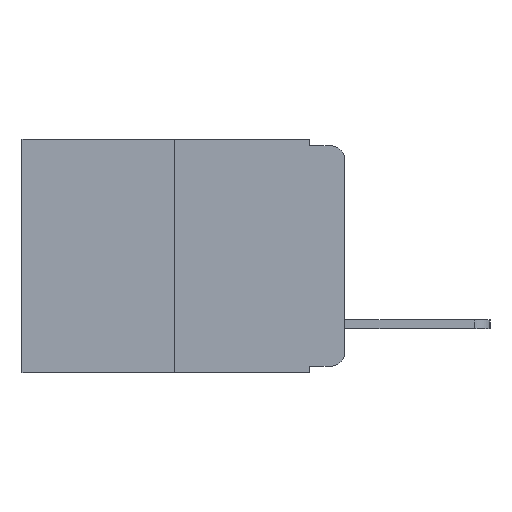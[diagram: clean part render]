
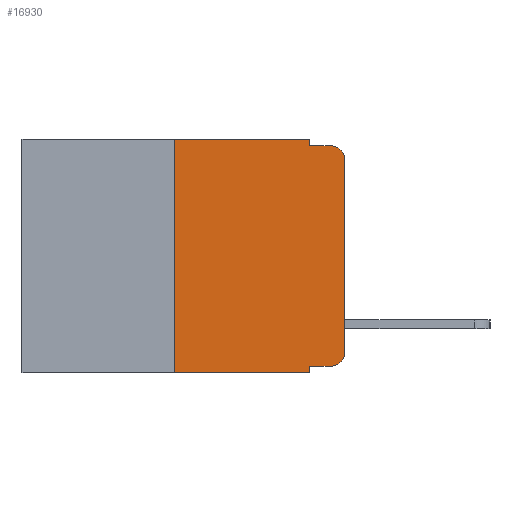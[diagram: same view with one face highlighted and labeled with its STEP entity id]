
A CAD part, left-side view. The second image highlights one B-rep face of the part: STEP entity #16930.
In plain terms, the highlighted planar face has unit normal (-1, 0, 0).
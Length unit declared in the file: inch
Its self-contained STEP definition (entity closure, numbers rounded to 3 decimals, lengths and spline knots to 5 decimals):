
#282 = ORIENTED_EDGE ( 'NONE', *, *, #3783, .F. ) ;
#1372 = DIRECTION ( 'NONE',  ( -1., 0., 0. ) ) ;
#2308 = VERTEX_POINT ( 'NONE', #12638 ) ;
#2593 = DIRECTION ( 'NONE',  ( 0., 0., -1. ) ) ;
#2771 = AXIS2_PLACEMENT_3D ( 'NONE', #6258, #17413, #7916 ) ;
#2850 = ORIENTED_EDGE ( 'NONE', *, *, #12250, .F. ) ;
#3260 = VECTOR ( 'NONE', #17030, 39.37008 ) ;
#3479 = DIRECTION ( 'NONE',  ( 0., -1., 0. ) ) ;
#3717 = CARTESIAN_POINT ( 'NONE',  ( 0., 0.051, 0. ) ) ;
#3783 = EDGE_CURVE ( 'NONE', #11301, #4717, #6162, .T. ) ;
#4101 = CIRCLE ( 'NONE', #8152, 0.02 ) ;
#4219 = CARTESIAN_POINT ( 'NONE',  ( 0., 0.051, -0.333 ) ) ;
#4538 = VECTOR ( 'NONE', #3479, 39.37008 ) ;
#4717 = VERTEX_POINT ( 'NONE', #18378 ) ;
#5120 = ORIENTED_EDGE ( 'NONE', *, *, #14346, .F. ) ;
#5604 = EDGE_CURVE ( 'NONE', #2308, #9613, #17796, .T. ) ;
#5658 = CARTESIAN_POINT ( 'NONE',  ( 0., 0.051, -0.01 ) ) ;
#5684 = CARTESIAN_POINT ( 'NONE',  ( 0., 0.051, 0. ) ) ;
#6162 = LINE ( 'NONE', #19746, #17871 ) ;
#6258 = CARTESIAN_POINT ( 'NONE',  ( 0., 0.02, -0.313 ) ) ;
#6442 = VERTEX_POINT ( 'NONE', #6681 ) ;
#6450 = LINE ( 'NONE', #9132, #6989 ) ;
#6535 = EDGE_LOOP ( 'NONE', ( #10719, #15408, #20553, #16887, #282, #5120, #18838, #2850, #7184, #16151 ) ) ;
#6622 = DIRECTION ( 'NONE',  ( 0., 0., 1. ) ) ;
#6681 = CARTESIAN_POINT ( 'NONE',  ( 0., 0.051, -0.333 ) ) ;
#6789 = CARTESIAN_POINT ( 'NONE',  ( 0., 0.051, -0.343 ) ) ;
#6989 = VECTOR ( 'NONE', #18608, 39.37008 ) ;
#7184 = ORIENTED_EDGE ( 'NONE', *, *, #11185, .T. ) ;
#7197 = CARTESIAN_POINT ( 'NONE',  ( 0., 0.473, -0.343 ) ) ;
#7211 = VERTEX_POINT ( 'NONE', #5658 ) ;
#7754 = VECTOR ( 'NONE', #14954, 39.37008 ) ;
#7916 = DIRECTION ( 'NONE',  ( 0., 0., -1. ) ) ;
#8152 = AXIS2_PLACEMENT_3D ( 'NONE', #11111, #1372, #12687 ) ;
#8579 = VECTOR ( 'NONE', #16921, 39.37008 ) ;
#9132 = CARTESIAN_POINT ( 'NONE',  ( 0., 0.051, -0.01 ) ) ;
#9613 = VERTEX_POINT ( 'NONE', #6789 ) ;
#10099 = EDGE_CURVE ( 'NONE', #15251, #13190, #12179, .T. ) ;
#10686 = CARTESIAN_POINT ( 'NONE',  ( 0., 0.473, 0. ) ) ;
#10719 = ORIENTED_EDGE ( 'NONE', *, *, #19610, .T. ) ;
#10966 = CARTESIAN_POINT ( 'NONE',  ( 0., 0.25, 0. ) ) ;
#11111 = CARTESIAN_POINT ( 'NONE',  ( 0., 0.02, -0.03 ) ) ;
#11185 = EDGE_CURVE ( 'NONE', #6442, #15251, #20222, .T. ) ;
#11301 = VERTEX_POINT ( 'NONE', #10966 ) ;
#12179 = CIRCLE ( 'NONE', #2771, 0.02 ) ;
#12250 = EDGE_CURVE ( 'NONE', #6442, #9613, #17518, .T. ) ;
#12296 = DIRECTION ( 'NONE',  ( 1., 0., 0. ) ) ;
#12573 = CARTESIAN_POINT ( 'NONE',  ( 0., 0.02, -0.01 ) ) ;
#12638 = CARTESIAN_POINT ( 'NONE',  ( 0., 0.25, -0.343 ) ) ;
#12687 = DIRECTION ( 'NONE',  ( 0., 0., -1. ) ) ;
#13190 = VERTEX_POINT ( 'NONE', #19416 ) ;
#13290 = EDGE_CURVE ( 'NONE', #4717, #7211, #16202, .T. ) ;
#13606 = CARTESIAN_POINT ( 'NONE',  ( 0., 0., -0.03 ) ) ;
#13790 = VECTOR ( 'NONE', #6622, 39.37008 ) ;
#14346 = EDGE_CURVE ( 'NONE', #2308, #11301, #20346, .T. ) ;
#14374 = DIRECTION ( 'NONE',  ( 0., 0., 1. ) ) ;
#14601 = CARTESIAN_POINT ( 'NONE',  ( 0., 0., 0. ) ) ;
#14704 = AXIS2_PLACEMENT_3D ( 'NONE', #10686, #12296, #2593 ) ;
#14954 = DIRECTION ( 'NONE',  ( 0., 0., -1. ) ) ;
#15251 = VERTEX_POINT ( 'NONE', #20105 ) ;
#15360 = VERTEX_POINT ( 'NONE', #12573 ) ;
#15402 = EDGE_CURVE ( 'NONE', #17376, #15360, #4101, .T. ) ;
#15408 = ORIENTED_EDGE ( 'NONE', *, *, #15402, .T. ) ;
#16151 = ORIENTED_EDGE ( 'NONE', *, *, #10099, .T. ) ;
#16183 = VECTOR ( 'NONE', #14374, 39.37008 ) ;
#16202 = LINE ( 'NONE', #3717, #7754 ) ;
#16887 = ORIENTED_EDGE ( 'NONE', *, *, #13290, .F. ) ;
#16921 = DIRECTION ( 'NONE',  ( 0., 0., -1. ) ) ;
#16930 = ADVANCED_FACE ( 'NONE', ( #17170 ), #16952, .F. ) ;
#16952 = PLANE ( 'NONE',  #14704 ) ;
#17030 = DIRECTION ( 'NONE',  ( 0., -1., 0. ) ) ;
#17170 = FACE_OUTER_BOUND ( 'NONE', #6535, .T. ) ;
#17376 = VERTEX_POINT ( 'NONE', #13606 ) ;
#17413 = DIRECTION ( 'NONE',  ( -1., 0., 0. ) ) ;
#17468 = CARTESIAN_POINT ( 'NONE',  ( 0., 0.25, 0. ) ) ;
#17510 = EDGE_CURVE ( 'NONE', #7211, #15360, #6450, .T. ) ;
#17518 = LINE ( 'NONE', #5684, #8579 ) ;
#17796 = LINE ( 'NONE', #7197, #4538 ) ;
#17871 = VECTOR ( 'NONE', #19727, 39.37008 ) ;
#17972 = LINE ( 'NONE', #14601, #13790 ) ;
#18378 = CARTESIAN_POINT ( 'NONE',  ( 0., 0.051, 0. ) ) ;
#18608 = DIRECTION ( 'NONE',  ( 0., -1., 0. ) ) ;
#18838 = ORIENTED_EDGE ( 'NONE', *, *, #5604, .T. ) ;
#19416 = CARTESIAN_POINT ( 'NONE',  ( 0., 0., -0.313 ) ) ;
#19610 = EDGE_CURVE ( 'NONE', #13190, #17376, #17972, .T. ) ;
#19727 = DIRECTION ( 'NONE',  ( 0., -1., 0. ) ) ;
#19746 = CARTESIAN_POINT ( 'NONE',  ( 0., 0.473, 0. ) ) ;
#20105 = CARTESIAN_POINT ( 'NONE',  ( 0., 0.02, -0.333 ) ) ;
#20222 = LINE ( 'NONE', #4219, #3260 ) ;
#20346 = LINE ( 'NONE', #17468, #16183 ) ;
#20553 = ORIENTED_EDGE ( 'NONE', *, *, #17510, .F. ) ;
